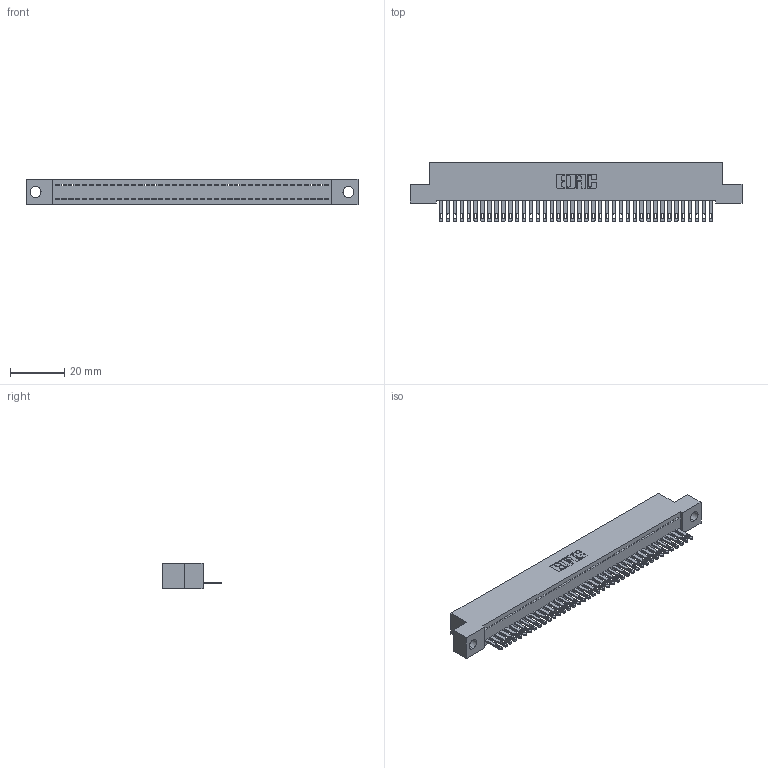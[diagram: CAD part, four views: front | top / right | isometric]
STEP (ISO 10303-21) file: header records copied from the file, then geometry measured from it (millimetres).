
FILE_DESCRIPTION (( 'STEP AP203' ), '1' );
FILE_NAME ('892-040-500-104.STEP', '2020-09-21T16:23:28', ( '' ), ( '' ), 'SwSTEP 2.0', 'SolidWorks 2020', '' );
FILE_SCHEMA (( 'CONFIG_CONTROL_DESIGN' ));
Length unit declared in the file: inch
Products named in the file (3): 842 Part_.156 TH; 892-040-500-104; 345-292-001_345-293-100
Assembly tree (41 placements, depth 2):
  892-040-500-104
    842 Part_.156 TH
    345-292-001_345-293-100  x40
Bounding box: 121.92 x 21.85 x 9.4 mm (x, y, z)
Volume: 10620.3 mm3; surface area: 15455.6 mm2
Topology: 41 solids, 41 shells, 2270 faces, 7019 edges, 4678 vertices
Faces by surface type: plane 1506, cylinder 764
Entity records: 24513 total; most frequent: CARTESIAN_POINT 4234, ORIENTED_EDGE 4210, DIRECTION 3577, EDGE_CURVE 2105, VECTOR 1973, LINE 1973, VERTEX_POINT 1402, AXIS2_PLACEMENT_3D 802
